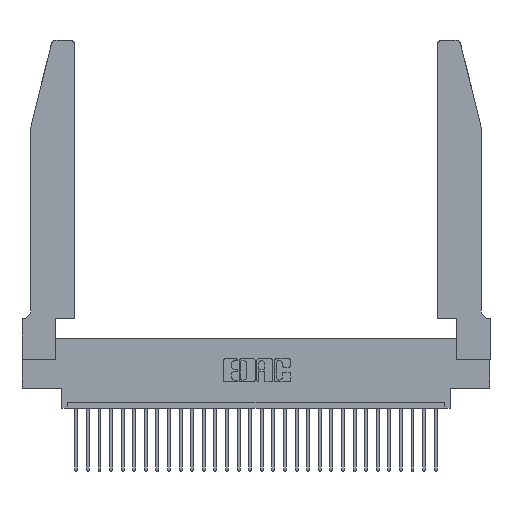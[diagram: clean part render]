
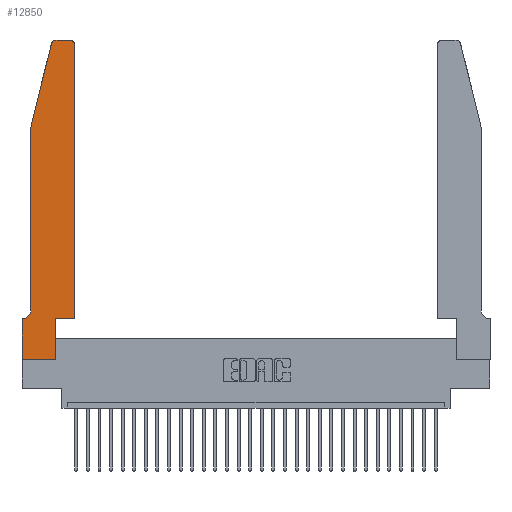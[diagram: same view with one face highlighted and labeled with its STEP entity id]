
A CAD part, top view. The second image highlights one B-rep face of the part: STEP entity #12850.
In plain terms, the highlighted planar face has unit normal (0, 0, 1).
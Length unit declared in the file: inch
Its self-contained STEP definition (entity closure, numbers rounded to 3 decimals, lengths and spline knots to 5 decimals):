
#34 = ORIENTED_EDGE ( 'NONE', *, *, #9576, .T. ) ;
#139 = DIRECTION ( 'NONE',  ( 1., 0., 0. ) ) ;
#333 = VECTOR ( 'NONE', #3050, 39.37008 ) ;
#1068 = LINE ( 'NONE', #23768, #333 ) ;
#1239 = VERTEX_POINT ( 'NONE', #11781 ) ;
#1412 = CARTESIAN_POINT ( 'NONE',  ( 0.284, 2.72, 0.37 ) ) ;
#1858 = VERTEX_POINT ( 'NONE', #8698 ) ;
#1951 = EDGE_CURVE ( 'NONE', #14281, #5118, #22819, .T. ) ;
#2176 = VECTOR ( 'NONE', #11527, 39.37008 ) ;
#3050 = DIRECTION ( 'NONE',  ( -1., 0., 0. ) ) ;
#3083 = ORIENTED_EDGE ( 'NONE', *, *, #12062, .T. ) ;
#3540 = VERTEX_POINT ( 'NONE', #25942 ) ;
#3696 = VECTOR ( 'NONE', #12535, 39.37008 ) ;
#3746 = DIRECTION ( 'NONE',  ( 0., 0., 1. ) ) ;
#4145 = EDGE_LOOP ( 'NONE', ( #16704, #6597, #28340, #34, #13718, #18549, #21589, #3083, #28300, #6224, #28037, #9385 ) ) ;
#4263 = EDGE_CURVE ( 'NONE', #4712, #3540, #12373, .T. ) ;
#4346 = EDGE_CURVE ( 'NONE', #1858, #18344, #27832, .T. ) ;
#4712 = VERTEX_POINT ( 'NONE', #9759 ) ;
#5118 = VERTEX_POINT ( 'NONE', #18446 ) ;
#5138 = LINE ( 'NONE', #5290, #3696 ) ;
#5192 = CARTESIAN_POINT ( 'NONE',  ( 0., 0.35, 0.37 ) ) ;
#5290 = CARTESIAN_POINT ( 'NONE',  ( 0.2605, 2.75, 0.37 ) ) ;
#5745 = LINE ( 'NONE', #11887, #15637 ) ;
#6224 = ORIENTED_EDGE ( 'NONE', *, *, #8776, .T. ) ;
#6597 = ORIENTED_EDGE ( 'NONE', *, *, #10039, .T. ) ;
#7415 = DIRECTION ( 'NONE',  ( 0., 0., 1. ) ) ;
#8247 = VERTEX_POINT ( 'NONE', #17212 ) ;
#8408 = DIRECTION ( 'NONE',  ( 1., 0., 0. ) ) ;
#8590 = DIRECTION ( 'NONE',  ( 0., 0., 1. ) ) ;
#8698 = CARTESIAN_POINT ( 'NONE',  ( 0., 0.35, 0.37 ) ) ;
#8776 = EDGE_CURVE ( 'NONE', #3540, #15735, #25279, .T. ) ;
#9152 = DIRECTION ( 'NONE',  ( 1., 0., 0. ) ) ;
#9385 = ORIENTED_EDGE ( 'NONE', *, *, #1951, .T. ) ;
#9413 = CARTESIAN_POINT ( 'NONE',  ( 0.0755, 2., 0.37 ) ) ;
#9416 = CARTESIAN_POINT ( 'NONE',  ( 0.0055, 0.42, 0.37 ) ) ;
#9459 = DIRECTION ( 'NONE',  ( 0., -1., 0. ) ) ;
#9576 = EDGE_CURVE ( 'NONE', #27704, #8247, #5745, .T. ) ;
#9759 = CARTESIAN_POINT ( 'NONE',  ( 0.2865, 0., 0.37 ) ) ;
#9867 = CIRCLE ( 'NONE', #22612, 0.07 ) ;
#10039 = EDGE_CURVE ( 'NONE', #1239, #30308, #27399, .T. ) ;
#11527 = DIRECTION ( 'NONE',  ( 0., 1., 0. ) ) ;
#11748 = DIRECTION ( 'NONE',  ( -1., 0., 0. ) ) ;
#11781 = CARTESIAN_POINT ( 'NONE',  ( 0.284, 2.75, 0.37 ) ) ;
#11887 = CARTESIAN_POINT ( 'NONE',  ( 0.0755, 2., 0.37 ) ) ;
#12062 = EDGE_CURVE ( 'NONE', #18344, #4712, #12594, .T. ) ;
#12373 = LINE ( 'NONE', #20927, #2176 ) ;
#12383 = CARTESIAN_POINT ( 'NONE',  ( 0.4505, 0.35, 0.37 ) ) ;
#12535 = DIRECTION ( 'NONE',  ( -1., 0., 0. ) ) ;
#12594 = LINE ( 'NONE', #20793, #24024 ) ;
#12850 = ADVANCED_FACE ( 'NONE', ( #13614 ), #16654, .T. ) ;
#13598 = VECTOR ( 'NONE', #16601, 39.37008 ) ;
#13614 = FACE_OUTER_BOUND ( 'NONE', #4145, .T. ) ;
#13718 = ORIENTED_EDGE ( 'NONE', *, *, #19876, .T. ) ;
#14110 = CARTESIAN_POINT ( 'NONE',  ( 0.4505, 0.35, 0.37 ) ) ;
#14127 = CARTESIAN_POINT ( 'NONE',  ( 0.4505, 0.35, 0.37 ) ) ;
#14281 = VERTEX_POINT ( 'NONE', #22615 ) ;
#14323 = CARTESIAN_POINT ( 'NONE',  ( 0.0055, 0.35, 0.37 ) ) ;
#15637 = VECTOR ( 'NONE', #9459, 39.37008 ) ;
#15735 = VERTEX_POINT ( 'NONE', #12383 ) ;
#16116 = VECTOR ( 'NONE', #21661, 39.37008 ) ;
#16601 = DIRECTION ( 'NONE',  ( 0., 1., 0. ) ) ;
#16654 = PLANE ( 'NONE',  #21117 ) ;
#16704 = ORIENTED_EDGE ( 'NONE', *, *, #28539, .T. ) ;
#17212 = CARTESIAN_POINT ( 'NONE',  ( 0.0755, 0.42, 0.37 ) ) ;
#17898 = VECTOR ( 'NONE', #23288, 39.37008 ) ;
#18344 = VERTEX_POINT ( 'NONE', #27937 ) ;
#18446 = CARTESIAN_POINT ( 'NONE',  ( 0.4205, 2.75, 0.37 ) ) ;
#18549 = ORIENTED_EDGE ( 'NONE', *, *, #25411, .T. ) ;
#18551 = CARTESIAN_POINT ( 'NONE',  ( 0.25487, 2.72718, 0.37 ) ) ;
#18727 = CARTESIAN_POINT ( 'NONE',  ( 0., 0., 0.37 ) ) ;
#19021 = VECTOR ( 'NONE', #139, 39.37008 ) ;
#19426 = EDGE_CURVE ( 'NONE', #30308, #27704, #27895, .T. ) ;
#19876 = EDGE_CURVE ( 'NONE', #8247, #29520, #9867, .T. ) ;
#20296 = AXIS2_PLACEMENT_3D ( 'NONE', #22889, #8590, #25045 ) ;
#20793 = CARTESIAN_POINT ( 'NONE',  ( 0., 0., 0.37 ) ) ;
#20927 = CARTESIAN_POINT ( 'NONE',  ( 0.2865, 0.35, 0.37 ) ) ;
#21117 = AXIS2_PLACEMENT_3D ( 'NONE', #5192, #7415, #23676 ) ;
#21358 = LINE ( 'NONE', #14127, #13598 ) ;
#21589 = ORIENTED_EDGE ( 'NONE', *, *, #4346, .T. ) ;
#21661 = DIRECTION ( 'NONE',  ( -0.239, -0.971, 0. ) ) ;
#22266 = EDGE_CURVE ( 'NONE', #15735, #14281, #21358, .T. ) ;
#22612 = AXIS2_PLACEMENT_3D ( 'NONE', #9416, #25850, #11748 ) ;
#22615 = CARTESIAN_POINT ( 'NONE',  ( 0.4505, 2.72, 0.37 ) ) ;
#22819 = CIRCLE ( 'NONE', #20296, 0.03 ) ;
#22889 = CARTESIAN_POINT ( 'NONE',  ( 0.4205, 2.72, 0.37 ) ) ;
#23288 = DIRECTION ( 'NONE',  ( 0., -1., 0. ) ) ;
#23676 = DIRECTION ( 'NONE',  ( 1., 0., 0. ) ) ;
#23768 = CARTESIAN_POINT ( 'NONE',  ( 0.0755, 0.35, 0.37 ) ) ;
#24024 = VECTOR ( 'NONE', #9152, 39.37008 ) ;
#25045 = DIRECTION ( 'NONE',  ( 1., 0., 0. ) ) ;
#25279 = LINE ( 'NONE', #14110, #19021 ) ;
#25374 = AXIS2_PLACEMENT_3D ( 'NONE', #1412, #3746, #8408 ) ;
#25411 = EDGE_CURVE ( 'NONE', #29520, #1858, #1068, .T. ) ;
#25850 = DIRECTION ( 'NONE',  ( 0., 0., -1. ) ) ;
#25942 = CARTESIAN_POINT ( 'NONE',  ( 0.2865, 0.35, 0.37 ) ) ;
#27399 = CIRCLE ( 'NONE', #25374, 0.03 ) ;
#27704 = VERTEX_POINT ( 'NONE', #9413 ) ;
#27832 = LINE ( 'NONE', #18727, #17898 ) ;
#27895 = LINE ( 'NONE', #28727, #16116 ) ;
#27937 = CARTESIAN_POINT ( 'NONE',  ( 0., 0., 0.37 ) ) ;
#28037 = ORIENTED_EDGE ( 'NONE', *, *, #22266, .T. ) ;
#28300 = ORIENTED_EDGE ( 'NONE', *, *, #4263, .T. ) ;
#28340 = ORIENTED_EDGE ( 'NONE', *, *, #19426, .T. ) ;
#28539 = EDGE_CURVE ( 'NONE', #5118, #1239, #5138, .T. ) ;
#28727 = CARTESIAN_POINT ( 'NONE',  ( 0.0755, 2., 0.37 ) ) ;
#29520 = VERTEX_POINT ( 'NONE', #14323 ) ;
#30308 = VERTEX_POINT ( 'NONE', #18551 ) ;
